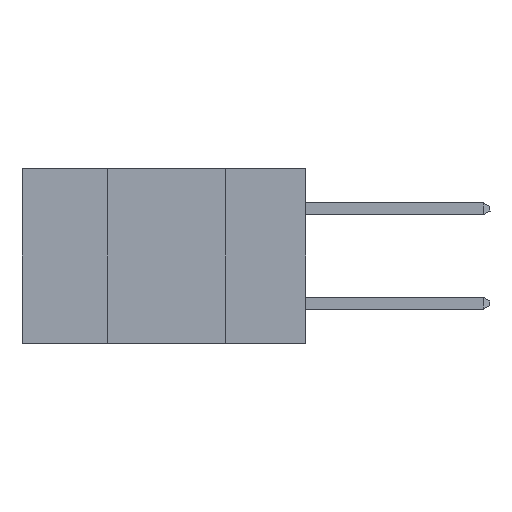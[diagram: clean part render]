
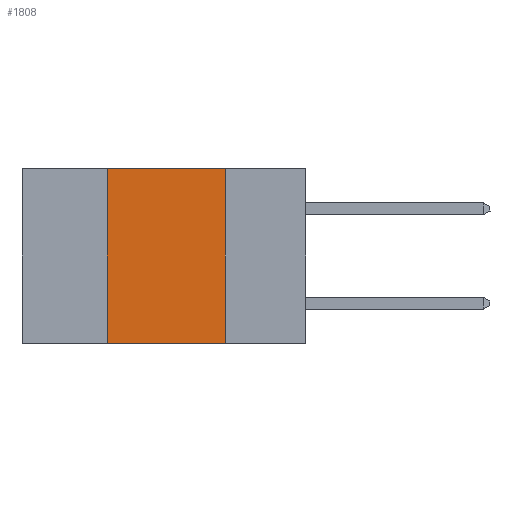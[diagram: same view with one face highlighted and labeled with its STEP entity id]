
A CAD part, left-side view. The second image highlights one B-rep face of the part: STEP entity #1808.
In plain terms, the highlighted planar face has unit normal (-1, 0, 0).
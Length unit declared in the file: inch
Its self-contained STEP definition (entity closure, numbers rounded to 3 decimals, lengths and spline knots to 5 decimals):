
#561 = CARTESIAN_POINT ( 'NONE',  ( 0., 0.6, 0. ) ) ;
#1808 = ADVANCED_FACE ( 'NONE', ( #9352 ), #15894, .F. ) ;
#2247 = DIRECTION ( 'NONE',  ( 0., -1., 0. ) ) ;
#2303 = CARTESIAN_POINT ( 'NONE',  ( 0., 0.6, -0.37 ) ) ;
#2480 = LINE ( 'NONE', #16466, #10533 ) ;
#2716 = VECTOR ( 'NONE', #2247, 39.37008 ) ;
#2764 = CARTESIAN_POINT ( 'NONE',  ( 0., 0.17, 0. ) ) ;
#4063 = CARTESIAN_POINT ( 'NONE',  ( 0., 0.17, -0.37 ) ) ;
#4346 = VERTEX_POINT ( 'NONE', #8389 ) ;
#5858 = VERTEX_POINT ( 'NONE', #4063 ) ;
#6631 = EDGE_CURVE ( 'NONE', #13493, #5858, #15534, .T. ) ;
#7314 = ORIENTED_EDGE ( 'NONE', *, *, #13649, .F. ) ;
#8389 = CARTESIAN_POINT ( 'NONE',  ( 0., 0.17, 0. ) ) ;
#8762 = DIRECTION ( 'NONE',  ( 0., 0., 1. ) ) ;
#8801 = VECTOR ( 'NONE', #9038, 39.37008 ) ;
#9038 = DIRECTION ( 'NONE',  ( 0., 0., -1. ) ) ;
#9352 = FACE_OUTER_BOUND ( 'NONE', #16013, .T. ) ;
#9556 = VERTEX_POINT ( 'NONE', #11400 ) ;
#9559 = VECTOR ( 'NONE', #11694, 39.37008 ) ;
#9819 = ORIENTED_EDGE ( 'NONE', *, *, #6631, .T. ) ;
#10533 = VECTOR ( 'NONE', #8762, 39.37008 ) ;
#10644 = CARTESIAN_POINT ( 'NONE',  ( 0., 0.6, 0. ) ) ;
#10823 = LINE ( 'NONE', #2764, #8801 ) ;
#11400 = CARTESIAN_POINT ( 'NONE',  ( 0., 0.42, 0. ) ) ;
#11694 = DIRECTION ( 'NONE',  ( 0., -1., 0. ) ) ;
#12161 = EDGE_CURVE ( 'NONE', #9556, #4346, #16183, .T. ) ;
#12793 = AXIS2_PLACEMENT_3D ( 'NONE', #561, #15943, #13446 ) ;
#13446 = DIRECTION ( 'NONE',  ( 0., 0., -1. ) ) ;
#13493 = VERTEX_POINT ( 'NONE', #14054 ) ;
#13649 = EDGE_CURVE ( 'NONE', #13493, #9556, #2480, .T. ) ;
#14054 = CARTESIAN_POINT ( 'NONE',  ( 0., 0.42, -0.37 ) ) ;
#15534 = LINE ( 'NONE', #2303, #2716 ) ;
#15894 = PLANE ( 'NONE',  #12793 ) ;
#15943 = DIRECTION ( 'NONE',  ( 1., 0., 0. ) ) ;
#16013 = EDGE_LOOP ( 'NONE', ( #16162, #16103, #7314, #9819 ) ) ;
#16103 = ORIENTED_EDGE ( 'NONE', *, *, #12161, .F. ) ;
#16162 = ORIENTED_EDGE ( 'NONE', *, *, #16509, .F. ) ;
#16183 = LINE ( 'NONE', #10644, #9559 ) ;
#16466 = CARTESIAN_POINT ( 'NONE',  ( 0., 0.42, 0. ) ) ;
#16509 = EDGE_CURVE ( 'NONE', #4346, #5858, #10823, .T. ) ;
